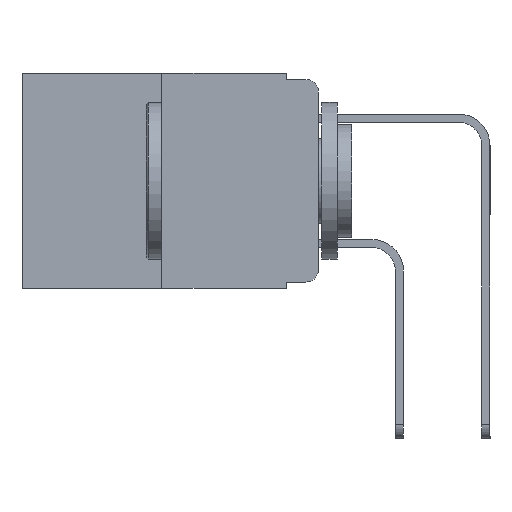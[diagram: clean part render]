
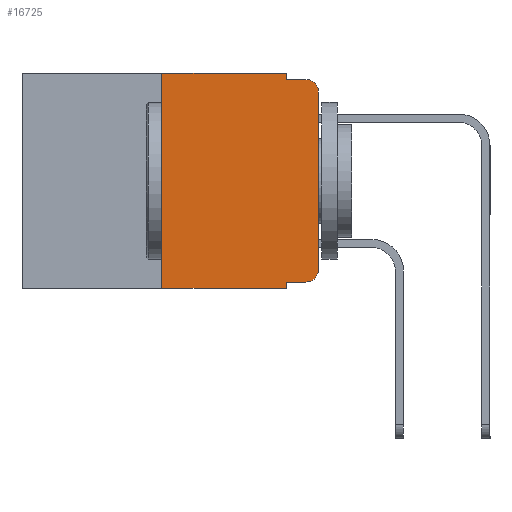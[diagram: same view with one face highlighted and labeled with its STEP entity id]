
A CAD part, left-side view. The second image highlights one B-rep face of the part: STEP entity #16725.
In plain terms, the highlighted planar face has unit normal (-1, 0, 0).
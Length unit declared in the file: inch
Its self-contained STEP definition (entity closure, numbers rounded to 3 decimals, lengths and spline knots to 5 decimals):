
#91 = VECTOR ( 'NONE', #2290, 39.37008 ) ;
#167 = ORIENTED_EDGE ( 'NONE', *, *, #3619, .T. ) ;
#252 = CARTESIAN_POINT ( 'NONE',  ( 0., 0.051, -0.343 ) ) ;
#588 = DIRECTION ( 'NONE',  ( 0., 0., -1. ) ) ;
#964 = VERTEX_POINT ( 'NONE', #14136 ) ;
#972 = CARTESIAN_POINT ( 'NONE',  ( 0., 0., -0.03 ) ) ;
#1265 = CARTESIAN_POINT ( 'NONE',  ( 0., 0.02, -0.313 ) ) ;
#1590 = VERTEX_POINT ( 'NONE', #6220 ) ;
#1745 = CARTESIAN_POINT ( 'NONE',  ( 0., 0.02, -0.01 ) ) ;
#1855 = EDGE_LOOP ( 'NONE', ( #16106, #16689, #2730, #8217, #3881, #14145, #167, #5604, #15279, #20587 ) ) ;
#2290 = DIRECTION ( 'NONE',  ( 0., -1., 0. ) ) ;
#2514 = LINE ( 'NONE', #20750, #21162 ) ;
#2730 = ORIENTED_EDGE ( 'NONE', *, *, #20295, .F. ) ;
#2805 = DIRECTION ( 'NONE',  ( 1., 0., 0. ) ) ;
#3099 = DIRECTION ( 'NONE',  ( 0., 0., -1. ) ) ;
#3619 = EDGE_CURVE ( 'NONE', #14855, #22435, #23146, .T. ) ;
#3881 = ORIENTED_EDGE ( 'NONE', *, *, #5167, .F. ) ;
#4566 = CIRCLE ( 'NONE', #5143, 0.02 ) ;
#5130 = DIRECTION ( 'NONE',  ( 0., -1., 0. ) ) ;
#5143 = AXIS2_PLACEMENT_3D ( 'NONE', #19029, #8276, #20826 ) ;
#5167 = EDGE_CURVE ( 'NONE', #21742, #16210, #22776, .T. ) ;
#5604 = ORIENTED_EDGE ( 'NONE', *, *, #16723, .F. ) ;
#5778 = CARTESIAN_POINT ( 'NONE',  ( 0., 0.473, 0. ) ) ;
#6114 = DIRECTION ( 'NONE',  ( 0., 0., 1. ) ) ;
#6220 = CARTESIAN_POINT ( 'NONE',  ( 0., 0., -0.313 ) ) ;
#6299 = LINE ( 'NONE', #9931, #15380 ) ;
#6335 = DIRECTION ( 'NONE',  ( 0., 0., -1. ) ) ;
#7226 = AXIS2_PLACEMENT_3D ( 'NONE', #20845, #2805, #15525 ) ;
#8217 = ORIENTED_EDGE ( 'NONE', *, *, #19078, .F. ) ;
#8276 = DIRECTION ( 'NONE',  ( -1., 0., 0. ) ) ;
#8293 = CARTESIAN_POINT ( 'NONE',  ( 0., 0.051, 0. ) ) ;
#9512 = EDGE_CURVE ( 'NONE', #964, #16896, #6299, .T. ) ;
#9519 = VECTOR ( 'NONE', #6335, 39.37008 ) ;
#9713 = CARTESIAN_POINT ( 'NONE',  ( 0., 0.25, -0.343 ) ) ;
#9931 = CARTESIAN_POINT ( 'NONE',  ( 0., 0.051, -0.333 ) ) ;
#9985 = CIRCLE ( 'NONE', #20306, 0.02 ) ;
#10063 = LINE ( 'NONE', #8293, #9519 ) ;
#11560 = CARTESIAN_POINT ( 'NONE',  ( 0., 0.051, 0. ) ) ;
#11902 = LINE ( 'NONE', #11560, #20844 ) ;
#11944 = PLANE ( 'NONE',  #7226 ) ;
#12175 = VERTEX_POINT ( 'NONE', #1745 ) ;
#12796 = VECTOR ( 'NONE', #6114, 39.37008 ) ;
#13709 = VECTOR ( 'NONE', #5130, 39.37008 ) ;
#14027 = DIRECTION ( 'NONE',  ( -1., 0., 0. ) ) ;
#14136 = CARTESIAN_POINT ( 'NONE',  ( 0., 0.051, -0.333 ) ) ;
#14145 = ORIENTED_EDGE ( 'NONE', *, *, #17901, .F. ) ;
#14207 = CARTESIAN_POINT ( 'NONE',  ( 0., 0.473, -0.343 ) ) ;
#14568 = VERTEX_POINT ( 'NONE', #23106 ) ;
#14855 = VERTEX_POINT ( 'NONE', #9713 ) ;
#15024 = CARTESIAN_POINT ( 'NONE',  ( 0., 0.051, -0.01 ) ) ;
#15279 = ORIENTED_EDGE ( 'NONE', *, *, #9512, .T. ) ;
#15380 = VECTOR ( 'NONE', #22599, 39.37008 ) ;
#15525 = DIRECTION ( 'NONE',  ( 0., 0., -1. ) ) ;
#16106 = ORIENTED_EDGE ( 'NONE', *, *, #22643, .T. ) ;
#16210 = VERTEX_POINT ( 'NONE', #19290 ) ;
#16689 = ORIENTED_EDGE ( 'NONE', *, *, #21465, .T. ) ;
#16723 = EDGE_CURVE ( 'NONE', #964, #22435, #10063, .T. ) ;
#16725 = ADVANCED_FACE ( 'NONE', ( #20147 ), #11944, .F. ) ;
#16896 = VERTEX_POINT ( 'NONE', #19589 ) ;
#17168 = DIRECTION ( 'NONE',  ( 0., 0., 1. ) ) ;
#17551 = LINE ( 'NONE', #18759, #12796 ) ;
#17901 = EDGE_CURVE ( 'NONE', #14855, #21742, #17551, .T. ) ;
#18759 = CARTESIAN_POINT ( 'NONE',  ( 0., 0.25, 0. ) ) ;
#18820 = LINE ( 'NONE', #15024, #91 ) ;
#19029 = CARTESIAN_POINT ( 'NONE',  ( 0., 0.02, -0.03 ) ) ;
#19078 = EDGE_CURVE ( 'NONE', #16210, #14568, #11902, .T. ) ;
#19290 = CARTESIAN_POINT ( 'NONE',  ( 0., 0.051, 0. ) ) ;
#19589 = CARTESIAN_POINT ( 'NONE',  ( 0., 0.02, -0.333 ) ) ;
#19717 = CARTESIAN_POINT ( 'NONE',  ( 0., 0.25, 0. ) ) ;
#20147 = FACE_OUTER_BOUND ( 'NONE', #1855, .T. ) ;
#20163 = DIRECTION ( 'NONE',  ( 0., -1., 0. ) ) ;
#20295 = EDGE_CURVE ( 'NONE', #14568, #12175, #18820, .T. ) ;
#20306 = AXIS2_PLACEMENT_3D ( 'NONE', #1265, #14027, #3099 ) ;
#20587 = ORIENTED_EDGE ( 'NONE', *, *, #22764, .T. ) ;
#20750 = CARTESIAN_POINT ( 'NONE',  ( 0., 0., 0. ) ) ;
#20826 = DIRECTION ( 'NONE',  ( 0., 0., -1. ) ) ;
#20844 = VECTOR ( 'NONE', #588, 39.37008 ) ;
#20845 = CARTESIAN_POINT ( 'NONE',  ( 0., 0.473, 0. ) ) ;
#21162 = VECTOR ( 'NONE', #17168, 39.37008 ) ;
#21465 = EDGE_CURVE ( 'NONE', #21483, #12175, #4566, .T. ) ;
#21483 = VERTEX_POINT ( 'NONE', #972 ) ;
#21742 = VERTEX_POINT ( 'NONE', #19717 ) ;
#22255 = VECTOR ( 'NONE', #20163, 39.37008 ) ;
#22435 = VERTEX_POINT ( 'NONE', #252 ) ;
#22599 = DIRECTION ( 'NONE',  ( 0., -1., 0. ) ) ;
#22643 = EDGE_CURVE ( 'NONE', #1590, #21483, #2514, .T. ) ;
#22764 = EDGE_CURVE ( 'NONE', #16896, #1590, #9985, .T. ) ;
#22776 = LINE ( 'NONE', #5778, #22255 ) ;
#23106 = CARTESIAN_POINT ( 'NONE',  ( 0., 0.051, -0.01 ) ) ;
#23146 = LINE ( 'NONE', #14207, #13709 ) ;
